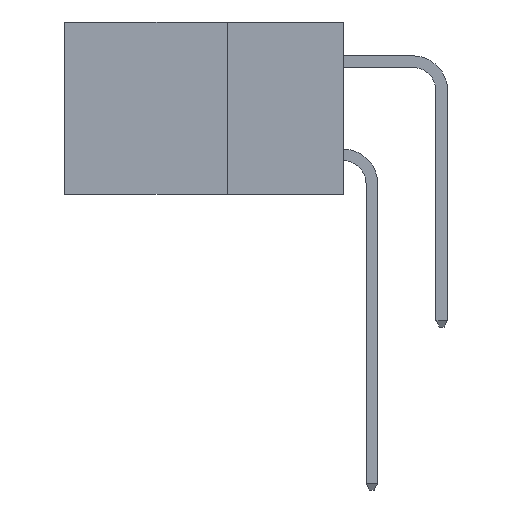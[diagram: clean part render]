
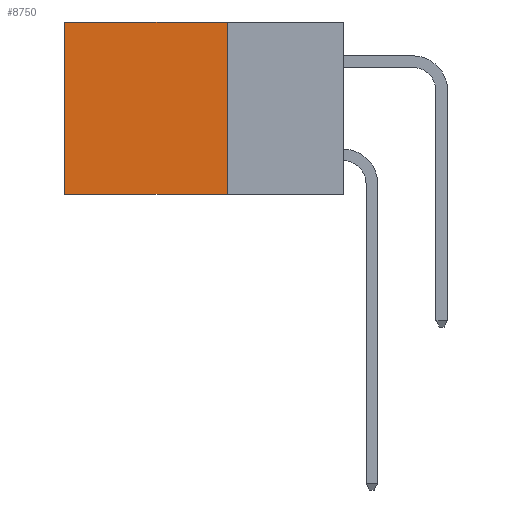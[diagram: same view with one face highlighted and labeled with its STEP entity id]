
A CAD part, left-side view. The second image highlights one B-rep face of the part: STEP entity #8750.
In plain terms, the highlighted planar face has unit normal (-1, 0, 0).
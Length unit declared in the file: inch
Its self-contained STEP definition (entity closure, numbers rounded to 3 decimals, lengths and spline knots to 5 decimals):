
#471 = CARTESIAN_POINT ( 'NONE',  ( 0.2615, 0.25, -0.37 ) ) ;
#572 = AXIS2_PLACEMENT_3D ( 'NONE', #3619, #4578, #10984 ) ;
#606 = EDGE_CURVE ( 'NONE', #3152, #8217, #3234, .T. ) ;
#1013 = CARTESIAN_POINT ( 'NONE',  ( 0.2615, 0.6, -0.37 ) ) ;
#1033 = ORIENTED_EDGE ( 'NONE', *, *, #8367, .T. ) ;
#2697 = PLANE ( 'NONE',  #572 ) ;
#3152 = VERTEX_POINT ( 'NONE', #11928 ) ;
#3227 = CARTESIAN_POINT ( 'NONE',  ( 0.2615, 0.25, 0. ) ) ;
#3234 = LINE ( 'NONE', #5391, #7908 ) ;
#3619 = CARTESIAN_POINT ( 'NONE',  ( 0.2615, 0.25, -0.37 ) ) ;
#4087 = EDGE_CURVE ( 'NONE', #8206, #5366, #6706, .T. ) ;
#4135 = VECTOR ( 'NONE', #5865, 39.37008 ) ;
#4442 = DIRECTION ( 'NONE',  ( 0., 0., -1. ) ) ;
#4578 = DIRECTION ( 'NONE',  ( 1., 0., 0. ) ) ;
#5366 = VERTEX_POINT ( 'NONE', #10054 ) ;
#5391 = CARTESIAN_POINT ( 'NONE',  ( 0.2615, 0.6, -0.37 ) ) ;
#5865 = DIRECTION ( 'NONE',  ( 0., 1., 0. ) ) ;
#6600 = EDGE_LOOP ( 'NONE', ( #8072, #8389, #7578, #1033 ) ) ;
#6706 = LINE ( 'NONE', #471, #8574 ) ;
#6800 = CARTESIAN_POINT ( 'NONE',  ( 0.2615, 0.25, -0.37 ) ) ;
#7401 = LINE ( 'NONE', #3227, #9246 ) ;
#7578 = ORIENTED_EDGE ( 'NONE', *, *, #4087, .F. ) ;
#7601 = CARTESIAN_POINT ( 'NONE',  ( 0.2615, 0.25, 0. ) ) ;
#7908 = VECTOR ( 'NONE', #4442, 39.37008 ) ;
#8072 = ORIENTED_EDGE ( 'NONE', *, *, #606, .T. ) ;
#8206 = VERTEX_POINT ( 'NONE', #7601 ) ;
#8217 = VERTEX_POINT ( 'NONE', #1013 ) ;
#8367 = EDGE_CURVE ( 'NONE', #8206, #3152, #7401, .T. ) ;
#8389 = ORIENTED_EDGE ( 'NONE', *, *, #10070, .F. ) ;
#8574 = VECTOR ( 'NONE', #8969, 39.37008 ) ;
#8750 = ADVANCED_FACE ( 'NONE', ( #10643 ), #2697, .F. ) ;
#8969 = DIRECTION ( 'NONE',  ( 0., 0., -1. ) ) ;
#9246 = VECTOR ( 'NONE', #9688, 39.37008 ) ;
#9688 = DIRECTION ( 'NONE',  ( 0., 1., 0. ) ) ;
#10054 = CARTESIAN_POINT ( 'NONE',  ( 0.2615, 0.25, -0.37 ) ) ;
#10070 = EDGE_CURVE ( 'NONE', #5366, #8217, #11459, .T. ) ;
#10643 = FACE_OUTER_BOUND ( 'NONE', #6600, .T. ) ;
#10984 = DIRECTION ( 'NONE',  ( 0., 0., -1. ) ) ;
#11459 = LINE ( 'NONE', #6800, #4135 ) ;
#11928 = CARTESIAN_POINT ( 'NONE',  ( 0.2615, 0.6, 0. ) ) ;
